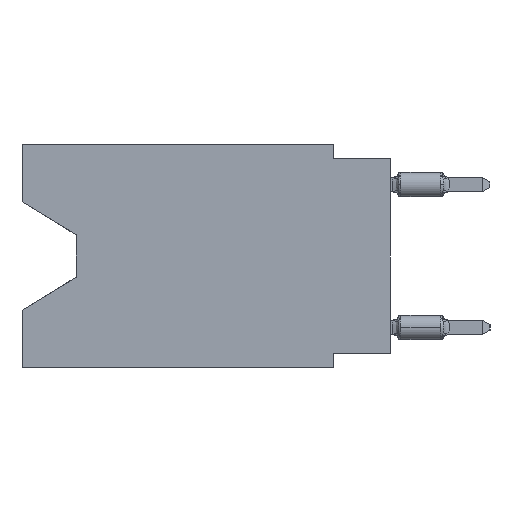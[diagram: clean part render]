
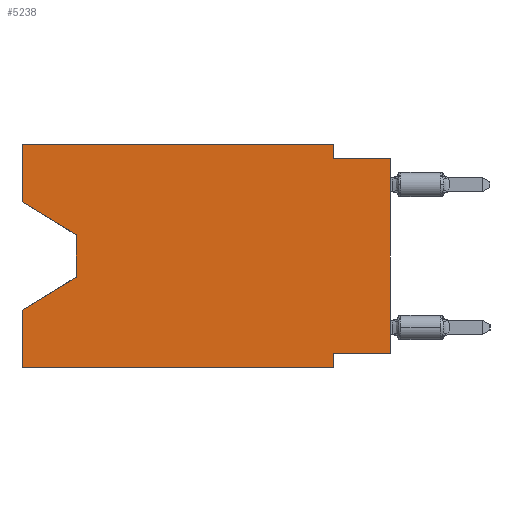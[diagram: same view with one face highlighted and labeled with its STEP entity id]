
A CAD part, left-side view. The second image highlights one B-rep face of the part: STEP entity #5238.
In plain terms, the highlighted planar face has unit normal (-1, 0, 0).
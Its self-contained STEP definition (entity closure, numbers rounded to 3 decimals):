
#138 = EDGE_CURVE ( 'NONE', #10123, #31660, #2874, .T. ) ;
#141 = VECTOR ( 'NONE', #12421, 1000. ) ;
#314 = LINE ( 'NONE', #17787, #20562 ) ;
#469 = EDGE_CURVE ( 'NONE', #11304, #31660, #18833, .T. ) ;
#846 = EDGE_CURVE ( 'NONE', #25026, #18986, #31957, .T. ) ;
#1314 = FACE_OUTER_BOUND ( 'NONE', #6969, .T. ) ;
#1432 = VERTEX_POINT ( 'NONE', #15227 ) ;
#2874 = LINE ( 'NONE', #24975, #141 ) ;
#3408 = CARTESIAN_POINT ( 'NONE',  ( 0., 2.54, -0.635 ) ) ;
#3433 = LINE ( 'NONE', #18253, #31511 ) ;
#3806 = LINE ( 'NONE', #5785, #31459 ) ;
#4007 = CARTESIAN_POINT ( 'NONE',  ( 0., 0., 0. ) ) ;
#4349 = CARTESIAN_POINT ( 'NONE',  ( 0., 13.97, -5.893 ) ) ;
#5238 = ADVANCED_FACE ( 'NONE', ( #1314 ), #32260, .F. ) ;
#5390 = CARTESIAN_POINT ( 'NONE',  ( 0., 2.54, 0. ) ) ;
#5785 = CARTESIAN_POINT ( 'NONE',  ( 0., 13.97, -4.013 ) ) ;
#6023 = CARTESIAN_POINT ( 'NONE',  ( 0., 0., -9.271 ) ) ;
#6574 = VERTEX_POINT ( 'NONE', #8905 ) ;
#6744 = CARTESIAN_POINT ( 'NONE',  ( 0., 16.383, -2.546 ) ) ;
#6886 = ORIENTED_EDGE ( 'NONE', *, *, #846, .F. ) ;
#6969 = EDGE_LOOP ( 'NONE', ( #13876, #13005, #22163, #6886, #7031, #13164, #11174, #11848, #21767, #28167, #7947, #22089 ) ) ;
#7031 = ORIENTED_EDGE ( 'NONE', *, *, #32453, .T. ) ;
#7224 = CARTESIAN_POINT ( 'NONE',  ( 0., 13.97, -5.893 ) ) ;
#7947 = ORIENTED_EDGE ( 'NONE', *, *, #29135, .F. ) ;
#8179 = CARTESIAN_POINT ( 'NONE',  ( 0., 0., -0.635 ) ) ;
#8905 = CARTESIAN_POINT ( 'NONE',  ( 0., 2.54, -9.906 ) ) ;
#9042 = DIRECTION ( 'NONE',  ( 0., 0., -1. ) ) ;
#10123 = VERTEX_POINT ( 'NONE', #3408 ) ;
#10215 = VERTEX_POINT ( 'NONE', #5390 ) ;
#11174 = ORIENTED_EDGE ( 'NONE', *, *, #12887, .F. ) ;
#11304 = VERTEX_POINT ( 'NONE', #26161 ) ;
#11848 = ORIENTED_EDGE ( 'NONE', *, *, #469, .T. ) ;
#12421 = DIRECTION ( 'NONE',  ( 0., -1., 0. ) ) ;
#12848 = CARTESIAN_POINT ( 'NONE',  ( 0., 16.383, 0. ) ) ;
#12887 = EDGE_CURVE ( 'NONE', #11304, #16037, #23977, .T. ) ;
#12975 = VERTEX_POINT ( 'NONE', #32387 ) ;
#13005 = ORIENTED_EDGE ( 'NONE', *, *, #13667, .T. ) ;
#13151 = CARTESIAN_POINT ( 'NONE',  ( 0., 2.54, 0. ) ) ;
#13164 = ORIENTED_EDGE ( 'NONE', *, *, #29668, .F. ) ;
#13667 = EDGE_CURVE ( 'NONE', #1432, #13808, #3806, .T. ) ;
#13808 = VERTEX_POINT ( 'NONE', #7224 ) ;
#13876 = ORIENTED_EDGE ( 'NONE', *, *, #18122, .T. ) ;
#14035 = LINE ( 'NONE', #4349, #29473 ) ;
#14105 = DIRECTION ( 'NONE',  ( 0., 0., 1. ) ) ;
#14120 = DIRECTION ( 'NONE',  ( 0., 0., -1. ) ) ;
#15227 = CARTESIAN_POINT ( 'NONE',  ( 0., 13.97, -4.013 ) ) ;
#15418 = CARTESIAN_POINT ( 'NONE',  ( 0., 16.383, -7.36 ) ) ;
#15474 = LINE ( 'NONE', #13151, #30001 ) ;
#16005 = VECTOR ( 'NONE', #27326, 1000. ) ;
#16037 = VERTEX_POINT ( 'NONE', #18481 ) ;
#16265 = LINE ( 'NONE', #21231, #28855 ) ;
#17075 = CARTESIAN_POINT ( 'NONE',  ( 0., 16.383, 0. ) ) ;
#17137 = DIRECTION ( 'NONE',  ( 0., 0., 1. ) ) ;
#17159 = LINE ( 'NONE', #12848, #20407 ) ;
#17787 = CARTESIAN_POINT ( 'NONE',  ( 0., 16.383, -2.546 ) ) ;
#18122 = EDGE_CURVE ( 'NONE', #21315, #1432, #314, .T. ) ;
#18253 = CARTESIAN_POINT ( 'NONE',  ( 0., 2.54, -9.906 ) ) ;
#18281 = DIRECTION ( 'NONE',  ( 0., -0.855, -0.519 ) ) ;
#18481 = CARTESIAN_POINT ( 'NONE',  ( 0., 2.54, -9.271 ) ) ;
#18833 = LINE ( 'NONE', #4007, #24953 ) ;
#18986 = VERTEX_POINT ( 'NONE', #15418 ) ;
#19193 = DIRECTION ( 'NONE',  ( 0., 1., 0. ) ) ;
#19411 = CARTESIAN_POINT ( 'NONE',  ( 0., 16.383, 0. ) ) ;
#20159 = CARTESIAN_POINT ( 'NONE',  ( 0., 16.383, -9.906 ) ) ;
#20407 = VECTOR ( 'NONE', #30337, 1000. ) ;
#20562 = VECTOR ( 'NONE', #18281, 1000. ) ;
#20618 = AXIS2_PLACEMENT_3D ( 'NONE', #17075, #31652, #9042 ) ;
#21033 = CARTESIAN_POINT ( 'NONE',  ( 0., 16.383, -9.906 ) ) ;
#21121 = VECTOR ( 'NONE', #19193, 1000. ) ;
#21231 = CARTESIAN_POINT ( 'NONE',  ( 0., 16.383, 0. ) ) ;
#21315 = VERTEX_POINT ( 'NONE', #6744 ) ;
#21759 = EDGE_CURVE ( 'NONE', #21315, #12975, #16265, .T. ) ;
#21767 = ORIENTED_EDGE ( 'NONE', *, *, #138, .F. ) ;
#22089 = ORIENTED_EDGE ( 'NONE', *, *, #21759, .F. ) ;
#22163 = ORIENTED_EDGE ( 'NONE', *, *, #23877, .T. ) ;
#23748 = DIRECTION ( 'NONE',  ( 0., 0., -1. ) ) ;
#23877 = EDGE_CURVE ( 'NONE', #13808, #18986, #14035, .T. ) ;
#23977 = LINE ( 'NONE', #6023, #21121 ) ;
#24109 = DIRECTION ( 'NONE',  ( 0., 0.855, -0.519 ) ) ;
#24624 = EDGE_CURVE ( 'NONE', #10215, #10123, #15474, .T. ) ;
#24953 = VECTOR ( 'NONE', #17137, 1000. ) ;
#24975 = CARTESIAN_POINT ( 'NONE',  ( 0., 0., -0.635 ) ) ;
#25026 = VERTEX_POINT ( 'NONE', #21033 ) ;
#26161 = CARTESIAN_POINT ( 'NONE',  ( 0., 0., -9.271 ) ) ;
#27098 = LINE ( 'NONE', #20159, #32334 ) ;
#27326 = DIRECTION ( 'NONE',  ( 0., 0., 1. ) ) ;
#28167 = ORIENTED_EDGE ( 'NONE', *, *, #24624, .F. ) ;
#28855 = VECTOR ( 'NONE', #14105, 1000. ) ;
#29135 = EDGE_CURVE ( 'NONE', #12975, #10215, #17159, .T. ) ;
#29473 = VECTOR ( 'NONE', #24109, 1000. ) ;
#29668 = EDGE_CURVE ( 'NONE', #16037, #6574, #3433, .T. ) ;
#30001 = VECTOR ( 'NONE', #14120, 1000. ) ;
#30216 = DIRECTION ( 'NONE',  ( 0., -1., 0. ) ) ;
#30337 = DIRECTION ( 'NONE',  ( 0., -1., 0. ) ) ;
#30459 = DIRECTION ( 'NONE',  ( 0., 0., -1. ) ) ;
#31459 = VECTOR ( 'NONE', #23748, 1000. ) ;
#31511 = VECTOR ( 'NONE', #30459, 1000. ) ;
#31652 = DIRECTION ( 'NONE',  ( 1., 0., 0. ) ) ;
#31660 = VERTEX_POINT ( 'NONE', #8179 ) ;
#31957 = LINE ( 'NONE', #19411, #16005 ) ;
#32260 = PLANE ( 'NONE',  #20618 ) ;
#32334 = VECTOR ( 'NONE', #30216, 1000. ) ;
#32387 = CARTESIAN_POINT ( 'NONE',  ( 0., 16.383, 0. ) ) ;
#32453 = EDGE_CURVE ( 'NONE', #25026, #6574, #27098, .T. ) ;
